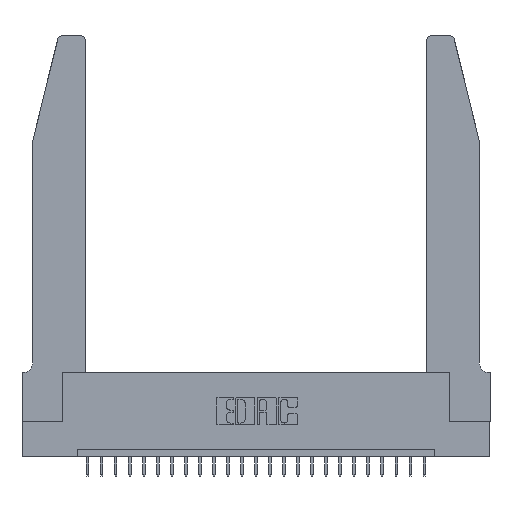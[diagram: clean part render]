
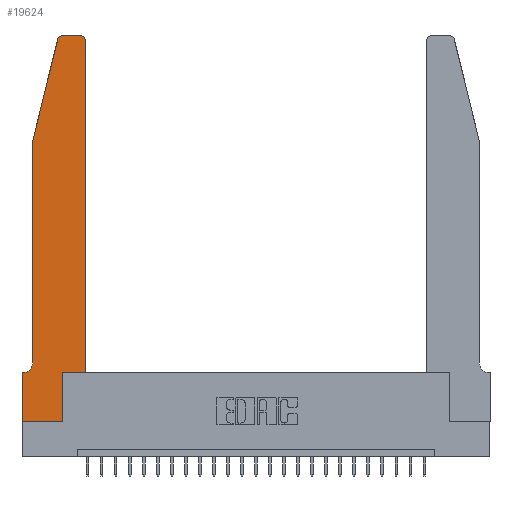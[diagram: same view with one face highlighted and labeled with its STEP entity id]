
A CAD part, top view. The second image highlights one B-rep face of the part: STEP entity #19624.
In plain terms, the highlighted planar face has unit normal (0, 0, 1).
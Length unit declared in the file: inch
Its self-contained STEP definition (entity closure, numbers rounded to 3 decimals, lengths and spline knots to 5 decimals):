
#245 = DIRECTION ( 'NONE',  ( 0., 0., -1. ) ) ;
#949 = LINE ( 'NONE', #11046, #17386 ) ;
#1094 = VERTEX_POINT ( 'NONE', #8293 ) ;
#1328 = DIRECTION ( 'NONE',  ( 0., 0., 1. ) ) ;
#1391 = CARTESIAN_POINT ( 'NONE',  ( 0.0755, 0.42, 0.37 ) ) ;
#1748 = VERTEX_POINT ( 'NONE', #9652 ) ;
#1758 = ORIENTED_EDGE ( 'NONE', *, *, #2268, .T. ) ;
#2185 = ORIENTED_EDGE ( 'NONE', *, *, #17644, .T. ) ;
#2232 = CARTESIAN_POINT ( 'NONE',  ( 0.284, 2.75, 0.37 ) ) ;
#2268 = EDGE_CURVE ( 'NONE', #13216, #25330, #16035, .T. ) ;
#2271 = DIRECTION ( 'NONE',  ( 0., 0., 1. ) ) ;
#2908 = VECTOR ( 'NONE', #13686, 39.37008 ) ;
#3707 = ORIENTED_EDGE ( 'NONE', *, *, #7487, .T. ) ;
#4152 = CARTESIAN_POINT ( 'NONE',  ( 0.4505, 0.35, 0.37 ) ) ;
#4200 = CARTESIAN_POINT ( 'NONE',  ( 0., 0.35, 0.37 ) ) ;
#4416 = CARTESIAN_POINT ( 'NONE',  ( 0.2865, 0., 0.37 ) ) ;
#4880 = DIRECTION ( 'NONE',  ( 0., 1., 0. ) ) ;
#5881 = LINE ( 'NONE', #23708, #13644 ) ;
#6112 = DIRECTION ( 'NONE',  ( 1., 0., 0. ) ) ;
#6440 = EDGE_CURVE ( 'NONE', #20939, #1094, #22790, .T. ) ;
#6506 = CARTESIAN_POINT ( 'NONE',  ( 0., 0., 0.37 ) ) ;
#6642 = EDGE_CURVE ( 'NONE', #1748, #18980, #22107, .T. ) ;
#6758 = ORIENTED_EDGE ( 'NONE', *, *, #19845, .T. ) ;
#7182 = EDGE_LOOP ( 'NONE', ( #18513, #25761, #3707, #14239, #14434, #2185, #7208, #8711, #21632, #8552, #1758, #6758 ) ) ;
#7208 = ORIENTED_EDGE ( 'NONE', *, *, #25259, .T. ) ;
#7274 = LINE ( 'NONE', #21290, #12906 ) ;
#7487 = EDGE_CURVE ( 'NONE', #1094, #15260, #5881, .T. ) ;
#7644 = CARTESIAN_POINT ( 'NONE',  ( 0.0755, 2., 0.37 ) ) ;
#7918 = DIRECTION ( 'NONE',  ( 0., 1., 0. ) ) ;
#8136 = CARTESIAN_POINT ( 'NONE',  ( 0.0755, 2., 0.37 ) ) ;
#8234 = AXIS2_PLACEMENT_3D ( 'NONE', #14308, #24765, #8303 ) ;
#8293 = CARTESIAN_POINT ( 'NONE',  ( 0.25487, 2.72718, 0.37 ) ) ;
#8303 = DIRECTION ( 'NONE',  ( 1., 0., 0. ) ) ;
#8552 = ORIENTED_EDGE ( 'NONE', *, *, #19391, .T. ) ;
#8711 = ORIENTED_EDGE ( 'NONE', *, *, #6642, .T. ) ;
#9015 = CARTESIAN_POINT ( 'NONE',  ( 0.4205, 2.75, 0.37 ) ) ;
#9108 = DIRECTION ( 'NONE',  ( 1., 0., 0. ) ) ;
#9652 = CARTESIAN_POINT ( 'NONE',  ( 0., 0., 0.37 ) ) ;
#9700 = CARTESIAN_POINT ( 'NONE',  ( 0.0755, 0.35, 0.37 ) ) ;
#9749 = LINE ( 'NONE', #7644, #2908 ) ;
#10419 = CIRCLE ( 'NONE', #24644, 0.07 ) ;
#10561 = DIRECTION ( 'NONE',  ( 1., 0., 0. ) ) ;
#11046 = CARTESIAN_POINT ( 'NONE',  ( 0.2865, 0.35, 0.37 ) ) ;
#11053 = CARTESIAN_POINT ( 'NONE',  ( 0.284, 2.72, 0.37 ) ) ;
#11137 = LINE ( 'NONE', #9700, #23592 ) ;
#11339 = DIRECTION ( 'NONE',  ( -1., 0., 0. ) ) ;
#11809 = DIRECTION ( 'NONE',  ( -1., 0., 0. ) ) ;
#11929 = VECTOR ( 'NONE', #18480, 39.37008 ) ;
#12283 = CARTESIAN_POINT ( 'NONE',  ( 0., 0.35, 0.37 ) ) ;
#12906 = VECTOR ( 'NONE', #11339, 39.37008 ) ;
#13215 = AXIS2_PLACEMENT_3D ( 'NONE', #11053, #1328, #9108 ) ;
#13216 = VERTEX_POINT ( 'NONE', #4152 ) ;
#13644 = VECTOR ( 'NONE', #17701, 39.37008 ) ;
#13686 = DIRECTION ( 'NONE',  ( 0., -1., 0. ) ) ;
#13821 = VERTEX_POINT ( 'NONE', #16878 ) ;
#13855 = PLANE ( 'NONE',  #17833 ) ;
#14239 = ORIENTED_EDGE ( 'NONE', *, *, #25429, .T. ) ;
#14308 = CARTESIAN_POINT ( 'NONE',  ( 0.4205, 2.72, 0.37 ) ) ;
#14434 = ORIENTED_EDGE ( 'NONE', *, *, #23589, .T. ) ;
#14869 = VECTOR ( 'NONE', #10561, 39.37008 ) ;
#15260 = VERTEX_POINT ( 'NONE', #8136 ) ;
#15299 = CARTESIAN_POINT ( 'NONE',  ( 0.0055, 0.35, 0.37 ) ) ;
#15478 = DIRECTION ( 'NONE',  ( -1., 0., 0. ) ) ;
#15653 = CARTESIAN_POINT ( 'NONE',  ( 0.4505, 0.35, 0.37 ) ) ;
#16035 = LINE ( 'NONE', #15653, #25238 ) ;
#16878 = CARTESIAN_POINT ( 'NONE',  ( 0.2865, 0.35, 0.37 ) ) ;
#16991 = CARTESIAN_POINT ( 'NONE',  ( 0.4505, 2.72, 0.37 ) ) ;
#17094 = EDGE_CURVE ( 'NONE', #18980, #13821, #949, .T. ) ;
#17386 = VECTOR ( 'NONE', #4880, 39.37008 ) ;
#17644 = EDGE_CURVE ( 'NONE', #25105, #21069, #11137, .T. ) ;
#17701 = DIRECTION ( 'NONE',  ( -0.239, -0.971, 0. ) ) ;
#17833 = AXIS2_PLACEMENT_3D ( 'NONE', #12283, #2271, #6112 ) ;
#18457 = VECTOR ( 'NONE', #21968, 39.37008 ) ;
#18480 = DIRECTION ( 'NONE',  ( 1., 0., 0. ) ) ;
#18513 = ORIENTED_EDGE ( 'NONE', *, *, #22401, .T. ) ;
#18867 = VERTEX_POINT ( 'NONE', #1391 ) ;
#18980 = VERTEX_POINT ( 'NONE', #4416 ) ;
#19177 = LINE ( 'NONE', #22245, #11929 ) ;
#19391 = EDGE_CURVE ( 'NONE', #13821, #13216, #19177, .T. ) ;
#19507 = CIRCLE ( 'NONE', #8234, 0.03 ) ;
#19624 = ADVANCED_FACE ( 'NONE', ( #22214 ), #13855, .T. ) ;
#19845 = EDGE_CURVE ( 'NONE', #25330, #20886, #19507, .T. ) ;
#19882 = CARTESIAN_POINT ( 'NONE',  ( 0., 0., 0.37 ) ) ;
#20886 = VERTEX_POINT ( 'NONE', #9015 ) ;
#20939 = VERTEX_POINT ( 'NONE', #2232 ) ;
#21069 = VERTEX_POINT ( 'NONE', #4200 ) ;
#21290 = CARTESIAN_POINT ( 'NONE',  ( 0.2605, 2.75, 0.37 ) ) ;
#21632 = ORIENTED_EDGE ( 'NONE', *, *, #17094, .T. ) ;
#21784 = CARTESIAN_POINT ( 'NONE',  ( 0.0055, 0.42, 0.37 ) ) ;
#21968 = DIRECTION ( 'NONE',  ( 0., -1., 0. ) ) ;
#22107 = LINE ( 'NONE', #6506, #14869 ) ;
#22214 = FACE_OUTER_BOUND ( 'NONE', #7182, .T. ) ;
#22245 = CARTESIAN_POINT ( 'NONE',  ( 0.4505, 0.35, 0.37 ) ) ;
#22401 = EDGE_CURVE ( 'NONE', #20886, #20939, #7274, .T. ) ;
#22461 = LINE ( 'NONE', #19882, #18457 ) ;
#22790 = CIRCLE ( 'NONE', #13215, 0.03 ) ;
#23589 = EDGE_CURVE ( 'NONE', #18867, #25105, #10419, .T. ) ;
#23592 = VECTOR ( 'NONE', #15478, 39.37008 ) ;
#23708 = CARTESIAN_POINT ( 'NONE',  ( 0.0755, 2., 0.37 ) ) ;
#24644 = AXIS2_PLACEMENT_3D ( 'NONE', #21784, #245, #11809 ) ;
#24765 = DIRECTION ( 'NONE',  ( 0., 0., 1. ) ) ;
#25105 = VERTEX_POINT ( 'NONE', #15299 ) ;
#25238 = VECTOR ( 'NONE', #7918, 39.37008 ) ;
#25259 = EDGE_CURVE ( 'NONE', #21069, #1748, #22461, .T. ) ;
#25330 = VERTEX_POINT ( 'NONE', #16991 ) ;
#25429 = EDGE_CURVE ( 'NONE', #15260, #18867, #9749, .T. ) ;
#25761 = ORIENTED_EDGE ( 'NONE', *, *, #6440, .T. ) ;
